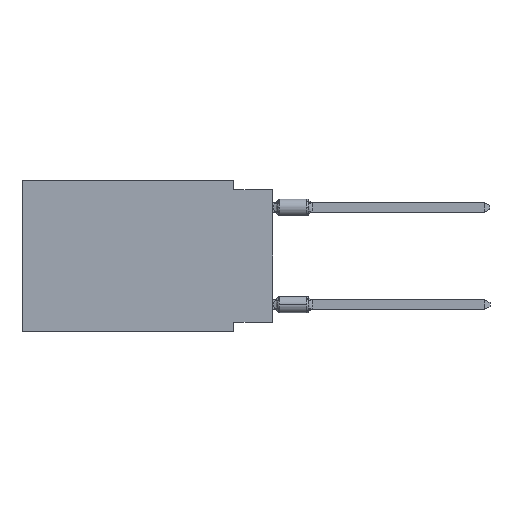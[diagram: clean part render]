
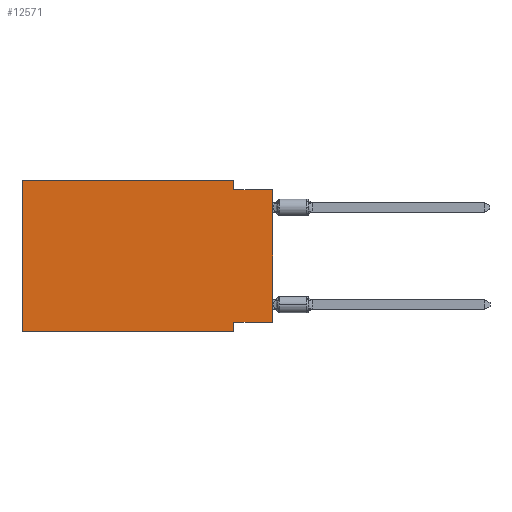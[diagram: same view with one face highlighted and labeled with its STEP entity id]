
A CAD part, left-side view. The second image highlights one B-rep face of the part: STEP entity #12571.
In plain terms, the highlighted planar face has unit normal (-1, 0, 0).
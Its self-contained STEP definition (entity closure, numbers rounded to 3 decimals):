
#209 = CARTESIAN_POINT ( 'NONE',  ( 0., 2.54, 0. ) ) ;
#808 = CARTESIAN_POINT ( 'NONE',  ( 0., 16.383, -9.906 ) ) ;
#1140 = FACE_OUTER_BOUND ( 'NONE', #8297, .T. ) ;
#1306 = CARTESIAN_POINT ( 'NONE',  ( 0., 0., -0.635 ) ) ;
#1407 = DIRECTION ( 'NONE',  ( 1., 0., 0. ) ) ;
#1566 = CARTESIAN_POINT ( 'NONE',  ( 0., 2.54, -0.635 ) ) ;
#2002 = CARTESIAN_POINT ( 'NONE',  ( 0., 0., -0.635 ) ) ;
#2048 = EDGE_CURVE ( 'NONE', #9266, #13273, #6010, .T. ) ;
#2716 = DIRECTION ( 'NONE',  ( 0., 0., -1. ) ) ;
#2720 = CARTESIAN_POINT ( 'NONE',  ( 0., 16.383, -9.906 ) ) ;
#2741 = VECTOR ( 'NONE', #11803, 1000. ) ;
#3196 = VECTOR ( 'NONE', #14381, 1000. ) ;
#3611 = ORIENTED_EDGE ( 'NONE', *, *, #11075, .F. ) ;
#3643 = CARTESIAN_POINT ( 'NONE',  ( 0., 2.54, -9.906 ) ) ;
#4058 = DIRECTION ( 'NONE',  ( 0., -1., 0. ) ) ;
#4169 = CARTESIAN_POINT ( 'NONE',  ( 0., 2.54, 0. ) ) ;
#4600 = LINE ( 'NONE', #14390, #4951 ) ;
#4884 = EDGE_CURVE ( 'NONE', #11135, #7974, #11983, .T. ) ;
#4951 = VECTOR ( 'NONE', #8668, 1000. ) ;
#5245 = VECTOR ( 'NONE', #4058, 1000. ) ;
#5262 = LINE ( 'NONE', #1306, #10310 ) ;
#6010 = LINE ( 'NONE', #10324, #7877 ) ;
#6405 = VERTEX_POINT ( 'NONE', #4169 ) ;
#6505 = CARTESIAN_POINT ( 'NONE',  ( 0., 16.383, 0. ) ) ;
#6682 = LINE ( 'NONE', #6505, #5245 ) ;
#6755 = VERTEX_POINT ( 'NONE', #9311 ) ;
#6826 = ORIENTED_EDGE ( 'NONE', *, *, #4884, .T. ) ;
#6906 = CARTESIAN_POINT ( 'NONE',  ( 0., 16.383, 0. ) ) ;
#7692 = CARTESIAN_POINT ( 'NONE',  ( 0., 0., -9.271 ) ) ;
#7877 = VECTOR ( 'NONE', #17302, 1000. ) ;
#7961 = DIRECTION ( 'NONE',  ( 0., 1., 0. ) ) ;
#7974 = VERTEX_POINT ( 'NONE', #2002 ) ;
#8224 = EDGE_CURVE ( 'NONE', #6755, #13571, #4600, .T. ) ;
#8297 = EDGE_LOOP ( 'NONE', ( #6826, #9339, #3611, #14364, #9342, #17516, #11975, #12013 ) ) ;
#8488 = EDGE_CURVE ( 'NONE', #9266, #13571, #17101, .T. ) ;
#8668 = DIRECTION ( 'NONE',  ( 0., 0., -1. ) ) ;
#8836 = VECTOR ( 'NONE', #15506, 1000. ) ;
#8993 = CARTESIAN_POINT ( 'NONE',  ( 0., 0., 0. ) ) ;
#9220 = VERTEX_POINT ( 'NONE', #1566 ) ;
#9266 = VERTEX_POINT ( 'NONE', #808 ) ;
#9311 = CARTESIAN_POINT ( 'NONE',  ( 0., 2.54, -9.271 ) ) ;
#9339 = ORIENTED_EDGE ( 'NONE', *, *, #12595, .F. ) ;
#9342 = ORIENTED_EDGE ( 'NONE', *, *, #2048, .F. ) ;
#10310 = VECTOR ( 'NONE', #18404, 1000. ) ;
#10324 = CARTESIAN_POINT ( 'NONE',  ( 0., 16.383, 0. ) ) ;
#10889 = VECTOR ( 'NONE', #7961, 1000. ) ;
#11071 = CARTESIAN_POINT ( 'NONE',  ( 0., 16.383, 0. ) ) ;
#11075 = EDGE_CURVE ( 'NONE', #6405, #9220, #17301, .T. ) ;
#11135 = VERTEX_POINT ( 'NONE', #14660 ) ;
#11803 = DIRECTION ( 'NONE',  ( 0., 0., 1. ) ) ;
#11975 = ORIENTED_EDGE ( 'NONE', *, *, #8224, .F. ) ;
#11983 = LINE ( 'NONE', #8993, #2741 ) ;
#12013 = ORIENTED_EDGE ( 'NONE', *, *, #12746, .F. ) ;
#12571 = ADVANCED_FACE ( 'NONE', ( #1140 ), #12580, .F. ) ;
#12580 = PLANE ( 'NONE',  #14815 ) ;
#12595 = EDGE_CURVE ( 'NONE', #9220, #7974, #5262, .T. ) ;
#12746 = EDGE_CURVE ( 'NONE', #11135, #6755, #16220, .T. ) ;
#13273 = VERTEX_POINT ( 'NONE', #6906 ) ;
#13571 = VERTEX_POINT ( 'NONE', #3643 ) ;
#14364 = ORIENTED_EDGE ( 'NONE', *, *, #18220, .F. ) ;
#14381 = DIRECTION ( 'NONE',  ( 0., 0., -1. ) ) ;
#14390 = CARTESIAN_POINT ( 'NONE',  ( 0., 2.54, -9.906 ) ) ;
#14660 = CARTESIAN_POINT ( 'NONE',  ( 0., 0., -9.271 ) ) ;
#14815 = AXIS2_PLACEMENT_3D ( 'NONE', #11071, #1407, #2716 ) ;
#15506 = DIRECTION ( 'NONE',  ( 0., -1., 0. ) ) ;
#16220 = LINE ( 'NONE', #7692, #10889 ) ;
#17101 = LINE ( 'NONE', #2720, #8836 ) ;
#17301 = LINE ( 'NONE', #209, #3196 ) ;
#17302 = DIRECTION ( 'NONE',  ( 0., 0., 1. ) ) ;
#17516 = ORIENTED_EDGE ( 'NONE', *, *, #8488, .T. ) ;
#18220 = EDGE_CURVE ( 'NONE', #13273, #6405, #6682, .T. ) ;
#18404 = DIRECTION ( 'NONE',  ( 0., -1., 0. ) ) ;
